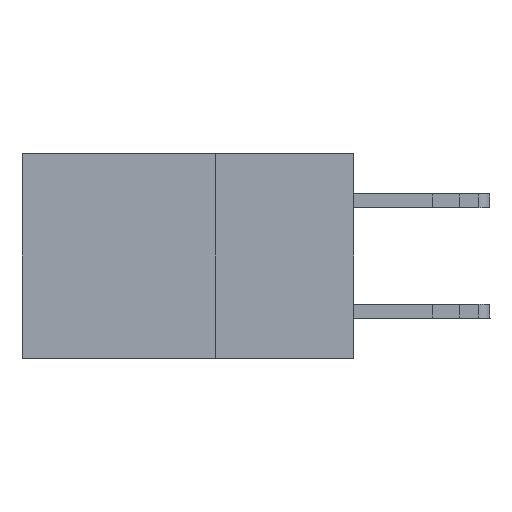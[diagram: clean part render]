
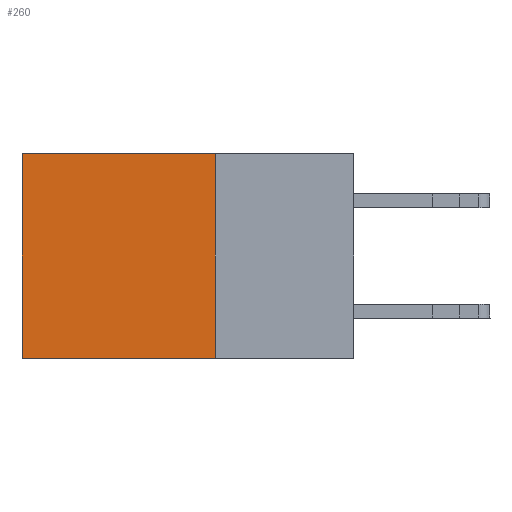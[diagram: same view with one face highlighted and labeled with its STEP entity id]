
A CAD part, left-side view. The second image highlights one B-rep face of the part: STEP entity #260.
In plain terms, the highlighted planar face has unit normal (-1, 0, 0).
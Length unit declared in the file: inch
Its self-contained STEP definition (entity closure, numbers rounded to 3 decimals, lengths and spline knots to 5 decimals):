
#260 = ADVANCED_FACE ( 'NONE', ( #6597 ), #21205, .F. ) ;
#501 = AXIS2_PLACEMENT_3D ( 'NONE', #20264, #20106, #20031 ) ;
#655 = ORIENTED_EDGE ( 'NONE', *, *, #23777, .F. ) ;
#1424 = LINE ( 'NONE', #20687, #15411 ) ;
#2396 = CARTESIAN_POINT ( 'NONE',  ( 0.2875, 0.25, 0. ) ) ;
#3835 = LINE ( 'NONE', #19693, #18263 ) ;
#3878 = EDGE_CURVE ( 'NONE', #11074, #17026, #1424, .T. ) ;
#3968 = DIRECTION ( 'NONE',  ( 0., 0., -1. ) ) ;
#5021 = VERTEX_POINT ( 'NONE', #2396 ) ;
#5033 = CARTESIAN_POINT ( 'NONE',  ( 0.2875, 0.25, 0. ) ) ;
#6597 = FACE_OUTER_BOUND ( 'NONE', #22676, .T. ) ;
#7162 = DIRECTION ( 'NONE',  ( 0., 1., 0. ) ) ;
#7284 = ORIENTED_EDGE ( 'NONE', *, *, #16002, .T. ) ;
#10866 = VECTOR ( 'NONE', #16356, 39.37008 ) ;
#11074 = VERTEX_POINT ( 'NONE', #21475 ) ;
#13353 = VECTOR ( 'NONE', #7162, 39.37008 ) ;
#13948 = LINE ( 'NONE', #21976, #13353 ) ;
#15015 = CARTESIAN_POINT ( 'NONE',  ( 0.2875, 0.25, -0.37 ) ) ;
#15113 = VERTEX_POINT ( 'NONE', #15015 ) ;
#15411 = VECTOR ( 'NONE', #3968, 39.37008 ) ;
#16002 = EDGE_CURVE ( 'NONE', #5021, #11074, #3835, .T. ) ;
#16356 = DIRECTION ( 'NONE',  ( 0., 0., -1. ) ) ;
#17026 = VERTEX_POINT ( 'NONE', #21851 ) ;
#18263 = VECTOR ( 'NONE', #21516, 39.37008 ) ;
#19517 = ORIENTED_EDGE ( 'NONE', *, *, #3878, .T. ) ;
#19693 = CARTESIAN_POINT ( 'NONE',  ( 0.2875, 0.25, 0. ) ) ;
#20031 = DIRECTION ( 'NONE',  ( 0., 0., -1. ) ) ;
#20106 = DIRECTION ( 'NONE',  ( 1., 0., 0. ) ) ;
#20264 = CARTESIAN_POINT ( 'NONE',  ( 0.2875, 0.25, 0. ) ) ;
#20560 = LINE ( 'NONE', #5033, #10866 ) ;
#20564 = EDGE_CURVE ( 'NONE', #15113, #17026, #13948, .T. ) ;
#20687 = CARTESIAN_POINT ( 'NONE',  ( 0.2875, 0.6, 0. ) ) ;
#21205 = PLANE ( 'NONE',  #501 ) ;
#21475 = CARTESIAN_POINT ( 'NONE',  ( 0.2875, 0.6, 0. ) ) ;
#21516 = DIRECTION ( 'NONE',  ( 0., 1., 0. ) ) ;
#21851 = CARTESIAN_POINT ( 'NONE',  ( 0.2875, 0.6, -0.37 ) ) ;
#21976 = CARTESIAN_POINT ( 'NONE',  ( 0.2875, 0.25, -0.37 ) ) ;
#22676 = EDGE_LOOP ( 'NONE', ( #19517, #23197, #655, #7284 ) ) ;
#23197 = ORIENTED_EDGE ( 'NONE', *, *, #20564, .F. ) ;
#23777 = EDGE_CURVE ( 'NONE', #5021, #15113, #20560, .T. ) ;
